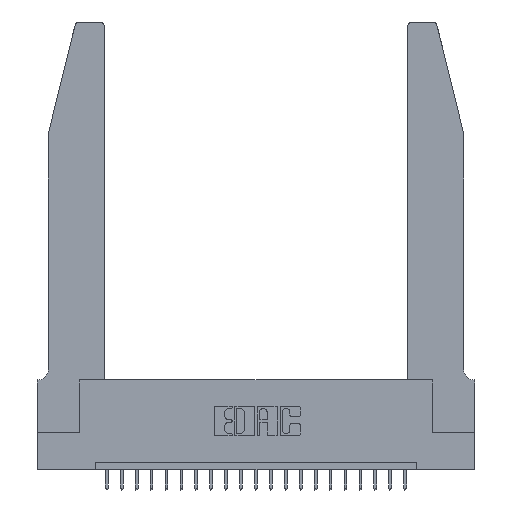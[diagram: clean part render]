
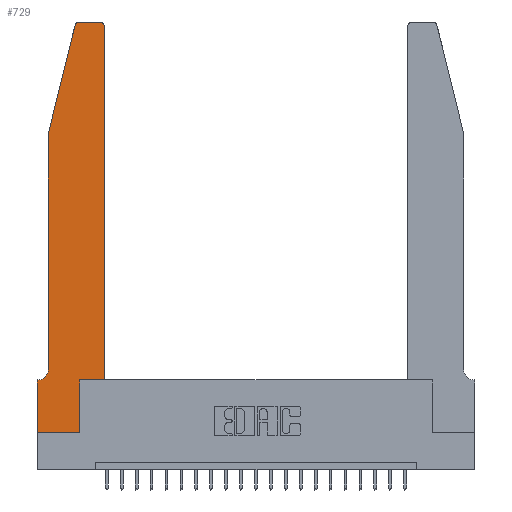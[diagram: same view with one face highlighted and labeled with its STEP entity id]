
A CAD part, top view. The second image highlights one B-rep face of the part: STEP entity #729.
In plain terms, the highlighted planar face has unit normal (0, 0, 1).
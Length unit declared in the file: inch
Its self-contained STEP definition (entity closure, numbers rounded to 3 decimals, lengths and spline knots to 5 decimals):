
#357 = AXIS2_PLACEMENT_3D ( 'NONE', #22397, #10878, #23302 ) ;
#459 = VERTEX_POINT ( 'NONE', #4889 ) ;
#649 = EDGE_CURVE ( 'NONE', #11238, #7547, #7998, .T. ) ;
#692 = LINE ( 'NONE', #9771, #7976 ) ;
#729 = ADVANCED_FACE ( 'NONE', ( #4503 ), #18931, .T. ) ;
#909 = VECTOR ( 'NONE', #4613, 39.37008 ) ;
#947 = DIRECTION ( 'NONE',  ( 0., 0., 1. ) ) ;
#989 = LINE ( 'NONE', #8264, #21840 ) ;
#1710 = CARTESIAN_POINT ( 'NONE',  ( 0.0055, 0.35, 0.37 ) ) ;
#2042 = VECTOR ( 'NONE', #12924, 39.37008 ) ;
#2596 = DIRECTION ( 'NONE',  ( -0.239, -0.971, 0. ) ) ;
#2660 = EDGE_CURVE ( 'NONE', #9804, #14052, #989, .T. ) ;
#2972 = DIRECTION ( 'NONE',  ( 1., 0., 0. ) ) ;
#3280 = ORIENTED_EDGE ( 'NONE', *, *, #21891, .T. ) ;
#3352 = CARTESIAN_POINT ( 'NONE',  ( 0.4505, 2.72, 0.37 ) ) ;
#4141 = LINE ( 'NONE', #18896, #15512 ) ;
#4144 = EDGE_CURVE ( 'NONE', #7459, #16362, #11165, .T. ) ;
#4444 = EDGE_CURVE ( 'NONE', #7547, #459, #18674, .T. ) ;
#4503 = FACE_OUTER_BOUND ( 'NONE', #21307, .T. ) ;
#4613 = DIRECTION ( 'NONE',  ( -1., 0., 0. ) ) ;
#4627 = VERTEX_POINT ( 'NONE', #3352 ) ;
#4650 = DIRECTION ( 'NONE',  ( -1., 0., 0. ) ) ;
#4889 = CARTESIAN_POINT ( 'NONE',  ( 0.25487, 2.72718, 0.37 ) ) ;
#5316 = CARTESIAN_POINT ( 'NONE',  ( 0.4205, 2.75, 0.37 ) ) ;
#5660 = CARTESIAN_POINT ( 'NONE',  ( 0.4505, 0.35, 0.37 ) ) ;
#6286 = CIRCLE ( 'NONE', #11601, 0.07 ) ;
#6562 = VERTEX_POINT ( 'NONE', #16469 ) ;
#6577 = ORIENTED_EDGE ( 'NONE', *, *, #23057, .T. ) ;
#6844 = LINE ( 'NONE', #19094, #23378 ) ;
#7159 = VERTEX_POINT ( 'NONE', #22017 ) ;
#7424 = CARTESIAN_POINT ( 'NONE',  ( 0.4505, 0.35, 0.37 ) ) ;
#7459 = VERTEX_POINT ( 'NONE', #15874 ) ;
#7547 = VERTEX_POINT ( 'NONE', #14889 ) ;
#7608 = CARTESIAN_POINT ( 'NONE',  ( 0., 0., 0.37 ) ) ;
#7976 = VECTOR ( 'NONE', #13055, 39.37008 ) ;
#7998 = LINE ( 'NONE', #19282, #909 ) ;
#8231 = CARTESIAN_POINT ( 'NONE',  ( 0., 0.35, 0.37 ) ) ;
#8264 = CARTESIAN_POINT ( 'NONE',  ( 0.0755, 0.35, 0.37 ) ) ;
#8397 = DIRECTION ( 'NONE',  ( 0., -1., 0. ) ) ;
#8402 = CARTESIAN_POINT ( 'NONE',  ( 0.2865, 0.35, 0.37 ) ) ;
#8577 = ORIENTED_EDGE ( 'NONE', *, *, #14587, .T. ) ;
#8879 = CARTESIAN_POINT ( 'NONE',  ( 0.284, 2.72, 0.37 ) ) ;
#9218 = ORIENTED_EDGE ( 'NONE', *, *, #13196, .T. ) ;
#9408 = LINE ( 'NONE', #5660, #2042 ) ;
#9771 = CARTESIAN_POINT ( 'NONE',  ( 0., 0., 0.37 ) ) ;
#9804 = VERTEX_POINT ( 'NONE', #1710 ) ;
#10287 = CARTESIAN_POINT ( 'NONE',  ( 0.0755, 0.42, 0.37 ) ) ;
#10710 = EDGE_CURVE ( 'NONE', #6562, #23476, #6844, .T. ) ;
#10878 = DIRECTION ( 'NONE',  ( 0., 0., 1. ) ) ;
#11076 = DIRECTION ( 'NONE',  ( -1., 0., 0. ) ) ;
#11165 = LINE ( 'NONE', #16834, #15998 ) ;
#11238 = VERTEX_POINT ( 'NONE', #5316 ) ;
#11601 = AXIS2_PLACEMENT_3D ( 'NONE', #19984, #21610, #11076 ) ;
#11606 = ORIENTED_EDGE ( 'NONE', *, *, #2660, .T. ) ;
#11927 = VECTOR ( 'NONE', #21600, 39.37008 ) ;
#12087 = EDGE_CURVE ( 'NONE', #7159, #14181, #19973, .T. ) ;
#12924 = DIRECTION ( 'NONE',  ( 0., 1., 0. ) ) ;
#13055 = DIRECTION ( 'NONE',  ( 0., -1., 0. ) ) ;
#13196 = EDGE_CURVE ( 'NONE', #459, #6562, #4141, .T. ) ;
#13221 = ORIENTED_EDGE ( 'NONE', *, *, #4444, .T. ) ;
#14052 = VERTEX_POINT ( 'NONE', #22182 ) ;
#14181 = VERTEX_POINT ( 'NONE', #20646 ) ;
#14468 = AXIS2_PLACEMENT_3D ( 'NONE', #8879, #15982, #23214 ) ;
#14587 = EDGE_CURVE ( 'NONE', #4627, #11238, #21977, .T. ) ;
#14889 = CARTESIAN_POINT ( 'NONE',  ( 0.284, 2.75, 0.37 ) ) ;
#14979 = AXIS2_PLACEMENT_3D ( 'NONE', #8231, #947, #2972 ) ;
#14999 = EDGE_CURVE ( 'NONE', #14052, #7159, #692, .T. ) ;
#15512 = VECTOR ( 'NONE', #2596, 39.37008 ) ;
#15874 = CARTESIAN_POINT ( 'NONE',  ( 0.2865, 0.35, 0.37 ) ) ;
#15982 = DIRECTION ( 'NONE',  ( 0., 0., 1. ) ) ;
#15998 = VECTOR ( 'NONE', #20067, 39.37008 ) ;
#16362 = VERTEX_POINT ( 'NONE', #7424 ) ;
#16469 = CARTESIAN_POINT ( 'NONE',  ( 0.0755, 2., 0.37 ) ) ;
#16834 = CARTESIAN_POINT ( 'NONE',  ( 0.4505, 0.35, 0.37 ) ) ;
#17088 = ORIENTED_EDGE ( 'NONE', *, *, #12087, .T. ) ;
#17984 = ORIENTED_EDGE ( 'NONE', *, *, #649, .T. ) ;
#18248 = EDGE_CURVE ( 'NONE', #14181, #7459, #18780, .T. ) ;
#18674 = CIRCLE ( 'NONE', #14468, 0.03 ) ;
#18780 = LINE ( 'NONE', #8402, #23176 ) ;
#18896 = CARTESIAN_POINT ( 'NONE',  ( 0.0755, 2., 0.37 ) ) ;
#18931 = PLANE ( 'NONE',  #14979 ) ;
#19094 = CARTESIAN_POINT ( 'NONE',  ( 0.0755, 2., 0.37 ) ) ;
#19282 = CARTESIAN_POINT ( 'NONE',  ( 0.2605, 2.75, 0.37 ) ) ;
#19685 = ORIENTED_EDGE ( 'NONE', *, *, #18248, .T. ) ;
#19973 = LINE ( 'NONE', #7608, #11927 ) ;
#19984 = CARTESIAN_POINT ( 'NONE',  ( 0.0055, 0.42, 0.37 ) ) ;
#20029 = ORIENTED_EDGE ( 'NONE', *, *, #10710, .T. ) ;
#20067 = DIRECTION ( 'NONE',  ( 1., 0., 0. ) ) ;
#20646 = CARTESIAN_POINT ( 'NONE',  ( 0.2865, 0., 0.37 ) ) ;
#20712 = ORIENTED_EDGE ( 'NONE', *, *, #4144, .T. ) ;
#20970 = DIRECTION ( 'NONE',  ( 0., 1., 0. ) ) ;
#21307 = EDGE_LOOP ( 'NONE', ( #17984, #13221, #9218, #20029, #6577, #11606, #21691, #17088, #19685, #20712, #3280, #8577 ) ) ;
#21600 = DIRECTION ( 'NONE',  ( 1., 0., 0. ) ) ;
#21610 = DIRECTION ( 'NONE',  ( 0., 0., -1. ) ) ;
#21691 = ORIENTED_EDGE ( 'NONE', *, *, #14999, .T. ) ;
#21840 = VECTOR ( 'NONE', #4650, 39.37008 ) ;
#21891 = EDGE_CURVE ( 'NONE', #16362, #4627, #9408, .T. ) ;
#21977 = CIRCLE ( 'NONE', #357, 0.03 ) ;
#22017 = CARTESIAN_POINT ( 'NONE',  ( 0., 0., 0.37 ) ) ;
#22182 = CARTESIAN_POINT ( 'NONE',  ( 0., 0.35, 0.37 ) ) ;
#22397 = CARTESIAN_POINT ( 'NONE',  ( 0.4205, 2.72, 0.37 ) ) ;
#23057 = EDGE_CURVE ( 'NONE', #23476, #9804, #6286, .T. ) ;
#23176 = VECTOR ( 'NONE', #20970, 39.37008 ) ;
#23214 = DIRECTION ( 'NONE',  ( 1., 0., 0. ) ) ;
#23302 = DIRECTION ( 'NONE',  ( 1., 0., 0. ) ) ;
#23378 = VECTOR ( 'NONE', #8397, 39.37008 ) ;
#23476 = VERTEX_POINT ( 'NONE', #10287 ) ;
